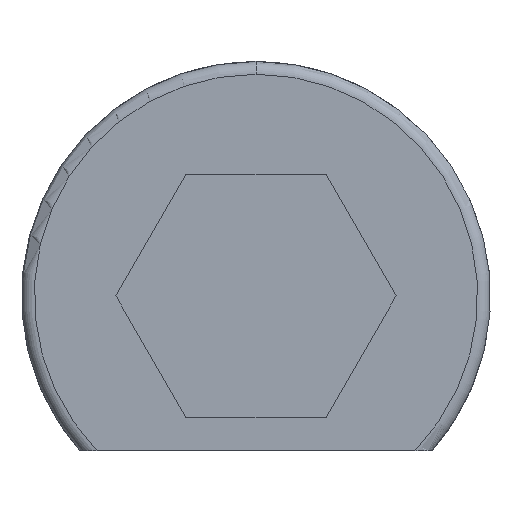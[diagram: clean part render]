
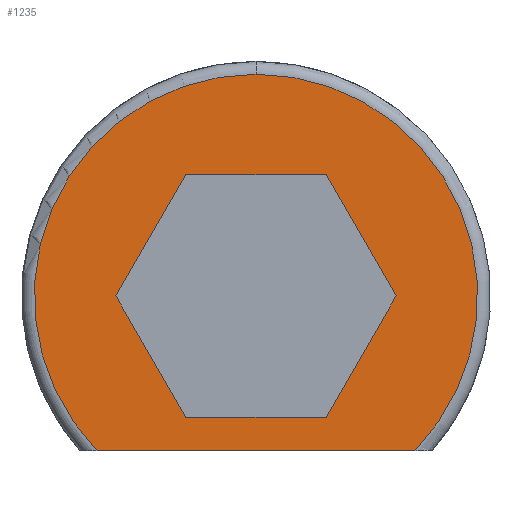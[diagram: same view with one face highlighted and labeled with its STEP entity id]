
A CAD part, left-side view. The second image highlights one B-rep face of the part: STEP entity #1235.
In plain terms, the highlighted planar face has unit normal (-1, 0, 0).
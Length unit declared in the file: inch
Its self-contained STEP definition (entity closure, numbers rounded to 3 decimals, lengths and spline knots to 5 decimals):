
#22 = VERTEX_POINT ( 'NONE', #1166 ) ;
#98 = ORIENTED_EDGE ( 'NONE', *, *, #2093, .F. ) ;
#148 = VERTEX_POINT ( 'NONE', #666 ) ;
#225 = EDGE_CURVE ( 'NONE', #2949, #148, #699, .T. ) ;
#245 = VERTEX_POINT ( 'NONE', #2977 ) ;
#262 = ORIENTED_EDGE ( 'NONE', *, *, #2213, .T. ) ;
#329 = DIRECTION ( 'NONE',  ( -1., 0., 0. ) ) ;
#343 = CIRCLE ( 'NONE', #1539, 0.26016 ) ;
#435 = CARTESIAN_POINT ( 'NONE',  ( 0., 0.16445, 0. ) ) ;
#483 = LINE ( 'NONE', #435, #3389 ) ;
#513 = ORIENTED_EDGE ( 'NONE', *, *, #822, .F. ) ;
#556 = LINE ( 'NONE', #690, #1787 ) ;
#666 = CARTESIAN_POINT ( 'NONE',  ( 0., 0.08223, 0.14242 ) ) ;
#667 = EDGE_LOOP ( 'NONE', ( #2057, #98, #513, #2925, #3206, #2907 ) ) ;
#690 = CARTESIAN_POINT ( 'NONE',  ( 0., 0.08223, -0.14242 ) ) ;
#699 = LINE ( 'NONE', #947, #2541 ) ;
#719 = DIRECTION ( 'NONE',  ( 0., 1., 0. ) ) ;
#817 = LINE ( 'NONE', #1720, #2442 ) ;
#822 = EDGE_CURVE ( 'NONE', #3514, #2121, #556, .T. ) ;
#829 = EDGE_CURVE ( 'NONE', #1942, #3514, #483, .T. ) ;
#858 = DIRECTION ( 'NONE',  ( 0., 0., 1. ) ) ;
#861 = CARTESIAN_POINT ( 'NONE',  ( 0., 0., 0.26016 ) ) ;
#878 = CARTESIAN_POINT ( 'NONE',  ( 0., -0.08223, 0.14242 ) ) ;
#900 = EDGE_CURVE ( 'NONE', #22, #2903, #343, .T. ) ;
#904 = VECTOR ( 'NONE', #3097, 39.37008 ) ;
#947 = CARTESIAN_POINT ( 'NONE',  ( 0., -0.08223, 0.14242 ) ) ;
#948 = EDGE_CURVE ( 'NONE', #148, #1942, #817, .T. ) ;
#975 = CARTESIAN_POINT ( 'NONE',  ( 0., 0.18652, -0.18136 ) ) ;
#1003 = VECTOR ( 'NONE', #1436, 39.37008 ) ;
#1040 = LINE ( 'NONE', #2557, #1003 ) ;
#1064 = CARTESIAN_POINT ( 'NONE',  ( 0., 0., 0.27516 ) ) ;
#1127 = DIRECTION ( 'NONE',  ( -1., 0., 0. ) ) ;
#1146 = DIRECTION ( 'NONE',  ( -1., 0., 0. ) ) ;
#1166 = CARTESIAN_POINT ( 'NONE',  ( 0., -0.18652, -0.18136 ) ) ;
#1235 = ADVANCED_FACE ( 'NONE', ( #1918, #3540 ), #1881, .T. ) ;
#1436 = DIRECTION ( 'NONE',  ( 0., 0.5, 0.866 ) ) ;
#1539 = AXIS2_PLACEMENT_3D ( 'NONE', #3474, #329, #1746 ) ;
#1617 = DIRECTION ( 'NONE',  ( 0., -0.5, -0.866 ) ) ;
#1655 = LINE ( 'NONE', #2503, #3219 ) ;
#1673 = AXIS2_PLACEMENT_3D ( 'NONE', #1064, #1146, #858 ) ;
#1720 = CARTESIAN_POINT ( 'NONE',  ( 0., 0.08223, 0.14242 ) ) ;
#1746 = DIRECTION ( 'NONE',  ( 0., 0., 1. ) ) ;
#1787 = VECTOR ( 'NONE', #3554, 39.37008 ) ;
#1871 = LINE ( 'NONE', #2761, #904 ) ;
#1881 = PLANE ( 'NONE',  #1673 ) ;
#1918 = FACE_BOUND ( 'NONE', #667, .T. ) ;
#1942 = VERTEX_POINT ( 'NONE', #3212 ) ;
#1962 = DIRECTION ( 'NONE',  ( 0., 1., 0. ) ) ;
#1977 = CARTESIAN_POINT ( 'NONE',  ( 0., 0.08223, -0.14242 ) ) ;
#2057 = ORIENTED_EDGE ( 'NONE', *, *, #2737, .F. ) ;
#2093 = EDGE_CURVE ( 'NONE', #2121, #245, #1871, .T. ) ;
#2121 = VERTEX_POINT ( 'NONE', #2751 ) ;
#2213 = EDGE_CURVE ( 'NONE', #2903, #2957, #2523, .T. ) ;
#2282 = ORIENTED_EDGE ( 'NONE', *, *, #3580, .F. ) ;
#2286 = DIRECTION ( 'NONE',  ( 0., 0., 1. ) ) ;
#2377 = ORIENTED_EDGE ( 'NONE', *, *, #900, .T. ) ;
#2442 = VECTOR ( 'NONE', #3143, 39.37008 ) ;
#2503 = CARTESIAN_POINT ( 'NONE',  ( 0., 0.20693, -0.18136 ) ) ;
#2523 = CIRCLE ( 'NONE', #2563, 0.26016 ) ;
#2541 = VECTOR ( 'NONE', #719, 39.37008 ) ;
#2557 = CARTESIAN_POINT ( 'NONE',  ( 0., -0.16445, 0. ) ) ;
#2563 = AXIS2_PLACEMENT_3D ( 'NONE', #2812, #1127, #2286 ) ;
#2737 = EDGE_CURVE ( 'NONE', #245, #2949, #1040, .T. ) ;
#2751 = CARTESIAN_POINT ( 'NONE',  ( 0., -0.08223, -0.14242 ) ) ;
#2761 = CARTESIAN_POINT ( 'NONE',  ( 0., -0.08223, -0.14242 ) ) ;
#2812 = CARTESIAN_POINT ( 'NONE',  ( 0., 0., 0. ) ) ;
#2903 = VERTEX_POINT ( 'NONE', #861 ) ;
#2907 = ORIENTED_EDGE ( 'NONE', *, *, #225, .F. ) ;
#2925 = ORIENTED_EDGE ( 'NONE', *, *, #829, .F. ) ;
#2949 = VERTEX_POINT ( 'NONE', #878 ) ;
#2957 = VERTEX_POINT ( 'NONE', #975 ) ;
#2977 = CARTESIAN_POINT ( 'NONE',  ( 0., -0.16445, 0. ) ) ;
#3097 = DIRECTION ( 'NONE',  ( 0., -0.5, 0.866 ) ) ;
#3143 = DIRECTION ( 'NONE',  ( 0., 0.5, -0.866 ) ) ;
#3206 = ORIENTED_EDGE ( 'NONE', *, *, #948, .F. ) ;
#3212 = CARTESIAN_POINT ( 'NONE',  ( 0., 0.16445, 0. ) ) ;
#3219 = VECTOR ( 'NONE', #1962, 39.37008 ) ;
#3389 = VECTOR ( 'NONE', #1617, 39.37008 ) ;
#3450 = EDGE_LOOP ( 'NONE', ( #2282, #2377, #262 ) ) ;
#3474 = CARTESIAN_POINT ( 'NONE',  ( 0., 0., 0. ) ) ;
#3514 = VERTEX_POINT ( 'NONE', #1977 ) ;
#3540 = FACE_OUTER_BOUND ( 'NONE', #3450, .T. ) ;
#3554 = DIRECTION ( 'NONE',  ( 0., -1., 0. ) ) ;
#3580 = EDGE_CURVE ( 'NONE', #22, #2957, #1655, .T. ) ;
